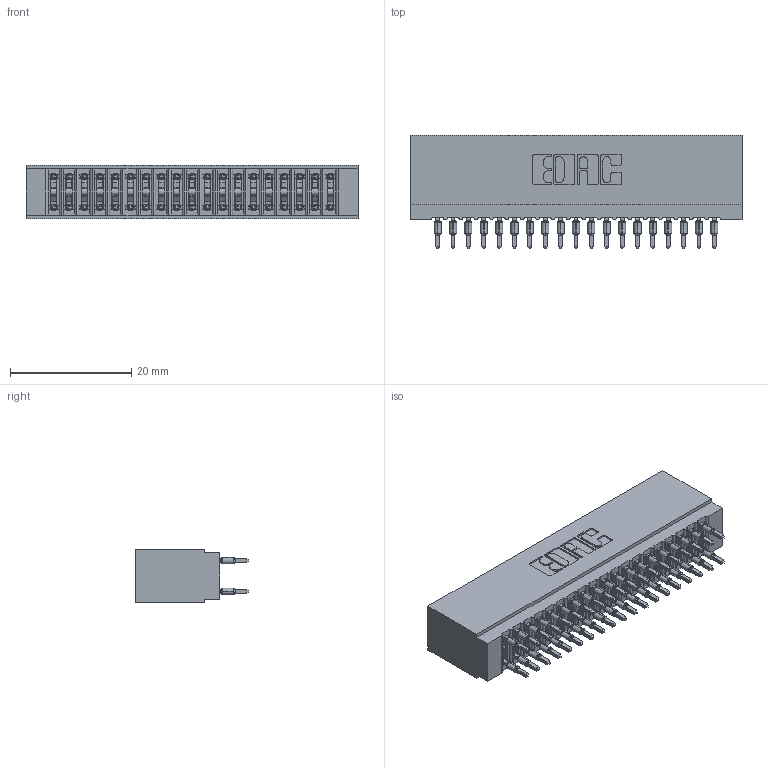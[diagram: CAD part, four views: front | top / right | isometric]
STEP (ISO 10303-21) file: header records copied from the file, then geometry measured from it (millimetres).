
FILE_DESCRIPTION (( 'STEP AP203' ), '1' );
FILE_NAME ('725-038-560-201.STEP', '2026-02-24T17:27:08', ( '' ), ( '' ), 'SwSTEP 2.0', 'SolidWorks 2023', '' );
FILE_SCHEMA (( 'CONFIG_CONTROL_DESIGN' ));
Length unit declared in the file: millimetre
Products named in the file (3): 745-292-001_560; 725-038-560-201; 725 Part_Insulator Option - 01
Assembly tree (39 placements, depth 2):
  725-038-560-201
    725 Part_Insulator Option - 01
    745-292-001_560  x38
Bounding box: 54.86 x 18.8 x 8.89 mm (x, y, z)
Volume: 4607 mm3; surface area: 9837.9 mm2
Topology: 39 solids, 39 shells, 3838 faces, 10495 edges, 6666 vertices
Faces by surface type: plane 1993, cylinder 857, bspline 760, torus 228
Entity records: 35414 total; most frequent: CARTESIAN_POINT 6653, ORIENTED_EDGE 6042, DIRECTION 5305, EDGE_CURVE 3021, VECTOR 2717, LINE 2717, VERTEX_POINT 1930, AXIS2_PLACEMENT_3D 1294
